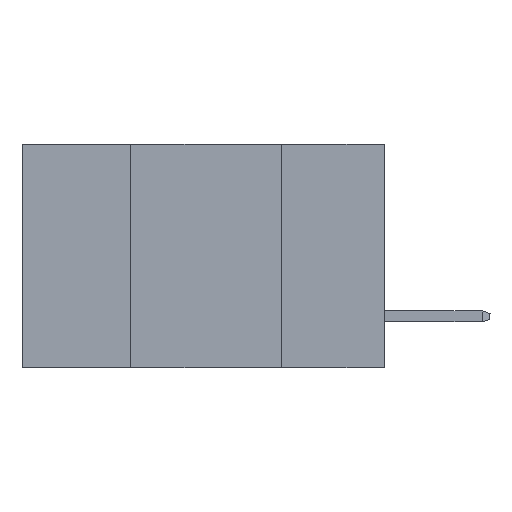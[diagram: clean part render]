
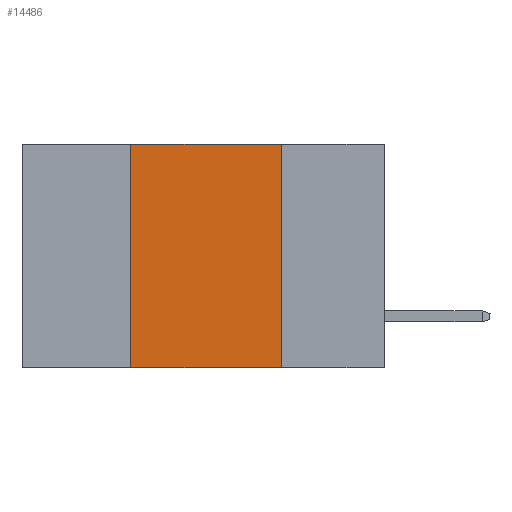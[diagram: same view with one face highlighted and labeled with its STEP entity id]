
A CAD part, left-side view. The second image highlights one B-rep face of the part: STEP entity #14486.
In plain terms, the highlighted planar face has unit normal (-1, 0, 0).
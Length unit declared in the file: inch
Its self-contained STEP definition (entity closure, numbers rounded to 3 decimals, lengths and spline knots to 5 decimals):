
#457 = VECTOR ( 'NONE', #13105, 39.37008 ) ;
#871 = AXIS2_PLACEMENT_3D ( 'NONE', #9952, #15760, #1237 ) ;
#983 = VERTEX_POINT ( 'NONE', #15222 ) ;
#1138 = PLANE ( 'NONE',  #871 ) ;
#1237 = DIRECTION ( 'NONE',  ( 0., 0., -1. ) ) ;
#1337 = LINE ( 'NONE', #7181, #457 ) ;
#1454 = CARTESIAN_POINT ( 'NONE',  ( 0., 0.17, -0.37 ) ) ;
#1521 = ORIENTED_EDGE ( 'NONE', *, *, #6346, .F. ) ;
#3222 = VECTOR ( 'NONE', #16429, 39.37008 ) ;
#3252 = LINE ( 'NONE', #8920, #3710 ) ;
#3499 = ORIENTED_EDGE ( 'NONE', *, *, #18380, .T. ) ;
#3710 = VECTOR ( 'NONE', #7676, 39.37008 ) ;
#3902 = CARTESIAN_POINT ( 'NONE',  ( 0., 0.17, -0.37 ) ) ;
#4023 = CARTESIAN_POINT ( 'NONE',  ( 0., 0.42, -0.37 ) ) ;
#4209 = LINE ( 'NONE', #1454, #14182 ) ;
#5983 = EDGE_CURVE ( 'NONE', #9154, #7284, #4209, .T. ) ;
#6346 = EDGE_CURVE ( 'NONE', #8276, #983, #1337, .T. ) ;
#7181 = CARTESIAN_POINT ( 'NONE',  ( 0., 0.42, -0.37 ) ) ;
#7284 = VERTEX_POINT ( 'NONE', #3902 ) ;
#7676 = DIRECTION ( 'NONE',  ( 0., -1., 0. ) ) ;
#8276 = VERTEX_POINT ( 'NONE', #4023 ) ;
#8903 = EDGE_CURVE ( 'NONE', #983, #9154, #17864, .T. ) ;
#8920 = CARTESIAN_POINT ( 'NONE',  ( 0., 0.6, -0.37 ) ) ;
#9154 = VERTEX_POINT ( 'NONE', #11369 ) ;
#9952 = CARTESIAN_POINT ( 'NONE',  ( 0., 0.6, 0. ) ) ;
#11369 = CARTESIAN_POINT ( 'NONE',  ( 0., 0.17, 0. ) ) ;
#11788 = DIRECTION ( 'NONE',  ( 0., 0., -1. ) ) ;
#12563 = ORIENTED_EDGE ( 'NONE', *, *, #8903, .F. ) ;
#13105 = DIRECTION ( 'NONE',  ( 0., 0., 1. ) ) ;
#14182 = VECTOR ( 'NONE', #11788, 39.37008 ) ;
#14233 = FACE_OUTER_BOUND ( 'NONE', #14265, .T. ) ;
#14265 = EDGE_LOOP ( 'NONE', ( #15336, #12563, #1521, #3499 ) ) ;
#14486 = ADVANCED_FACE ( 'NONE', ( #14233 ), #1138, .F. ) ;
#15222 = CARTESIAN_POINT ( 'NONE',  ( 0., 0.42, 0. ) ) ;
#15336 = ORIENTED_EDGE ( 'NONE', *, *, #5983, .F. ) ;
#15760 = DIRECTION ( 'NONE',  ( 1., 0., 0. ) ) ;
#16429 = DIRECTION ( 'NONE',  ( 0., -1., 0. ) ) ;
#16620 = CARTESIAN_POINT ( 'NONE',  ( 0., 0.6, 0. ) ) ;
#17864 = LINE ( 'NONE', #16620, #3222 ) ;
#18380 = EDGE_CURVE ( 'NONE', #8276, #7284, #3252, .T. ) ;
